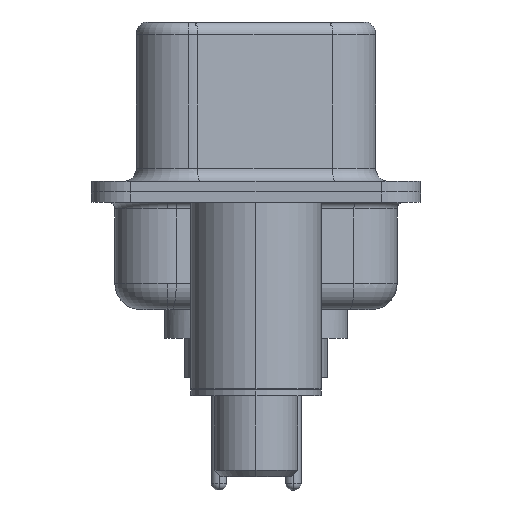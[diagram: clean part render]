
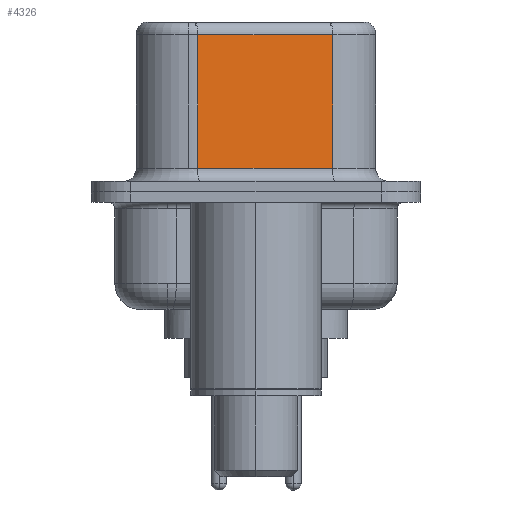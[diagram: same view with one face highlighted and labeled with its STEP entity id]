
A CAD part, left-side view. The second image highlights one B-rep face of the part: STEP entity #4326.
In plain terms, the highlighted planar face has unit normal (-0.985, -0.174, 0).
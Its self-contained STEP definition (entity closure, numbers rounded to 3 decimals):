
#281 = EDGE_LOOP ( 'NONE', ( #19551, #21884, #7215, #4545 ) ) ;
#4326 = ADVANCED_FACE ( 'NONE', ( #12212 ), #17947, .F. ) ;
#4545 = ORIENTED_EDGE ( 'NONE', *, *, #15342, .T. ) ;
#4576 = LINE ( 'NONE', #8426, #20915 ) ;
#4860 = LINE ( 'NONE', #10001, #16184 ) ;
#5851 = DIRECTION ( 'NONE',  ( 0.174, -0.985, 0. ) ) ;
#6793 = VECTOR ( 'NONE', #9527, 1000. ) ;
#7085 = DIRECTION ( 'NONE',  ( -0.174, 0.985, 0. ) ) ;
#7159 = CARTESIAN_POINT ( 'NONE',  ( 3.67, 2.233, 0.9 ) ) ;
#7215 = ORIENTED_EDGE ( 'NONE', *, *, #25720, .T. ) ;
#8065 = VERTEX_POINT ( 'NONE', #7159 ) ;
#8426 = CARTESIAN_POINT ( 'NONE',  ( 3.67, 2.233, 6.52 ) ) ;
#9527 = DIRECTION ( 'NONE',  ( 0., 0., -1. ) ) ;
#9931 = VERTEX_POINT ( 'NONE', #15710 ) ;
#10001 = CARTESIAN_POINT ( 'NONE',  ( 4.58, -2.927, 0.9 ) ) ;
#10538 = AXIS2_PLACEMENT_3D ( 'NONE', #20104, #17956, #15798 ) ;
#12212 = FACE_OUTER_BOUND ( 'NONE', #281, .T. ) ;
#13066 = LINE ( 'NONE', #24412, #6793 ) ;
#15031 = VECTOR ( 'NONE', #7085, 1000. ) ;
#15076 = CARTESIAN_POINT ( 'NONE',  ( 4.58, -2.927, 6.02 ) ) ;
#15342 = EDGE_CURVE ( 'NONE', #8065, #23125, #4860, .T. ) ;
#15527 = CARTESIAN_POINT ( 'NONE',  ( 4.58, -2.927, 6.02 ) ) ;
#15710 = CARTESIAN_POINT ( 'NONE',  ( 3.67, 2.233, 6.02 ) ) ;
#15798 = DIRECTION ( 'NONE',  ( -0.174, 0.985, 0. ) ) ;
#16184 = VECTOR ( 'NONE', #5851, 1000. ) ;
#16381 = EDGE_CURVE ( 'NONE', #20481, #23125, #13066, .T. ) ;
#17844 = EDGE_CURVE ( 'NONE', #20481, #9931, #22071, .T. ) ;
#17947 = PLANE ( 'NONE',  #10538 ) ;
#17956 = DIRECTION ( 'NONE',  ( 0.985, 0.174, 0. ) ) ;
#19166 = CARTESIAN_POINT ( 'NONE',  ( 4.58, -2.927, 0.9 ) ) ;
#19551 = ORIENTED_EDGE ( 'NONE', *, *, #16381, .F. ) ;
#20104 = CARTESIAN_POINT ( 'NONE',  ( 4.58, -2.927, 6.52 ) ) ;
#20481 = VERTEX_POINT ( 'NONE', #15076 ) ;
#20915 = VECTOR ( 'NONE', #23303, 1000. ) ;
#21884 = ORIENTED_EDGE ( 'NONE', *, *, #17844, .T. ) ;
#22071 = LINE ( 'NONE', #15527, #15031 ) ;
#23125 = VERTEX_POINT ( 'NONE', #19166 ) ;
#23303 = DIRECTION ( 'NONE',  ( 0., 0., -1. ) ) ;
#24412 = CARTESIAN_POINT ( 'NONE',  ( 4.58, -2.927, 6.52 ) ) ;
#25720 = EDGE_CURVE ( 'NONE', #9931, #8065, #4576, .T. ) ;
